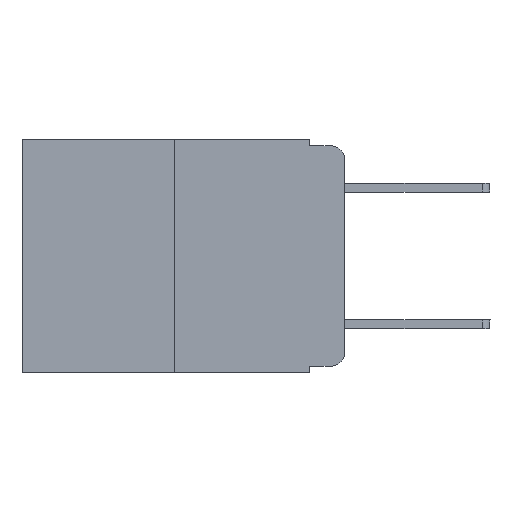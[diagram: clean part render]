
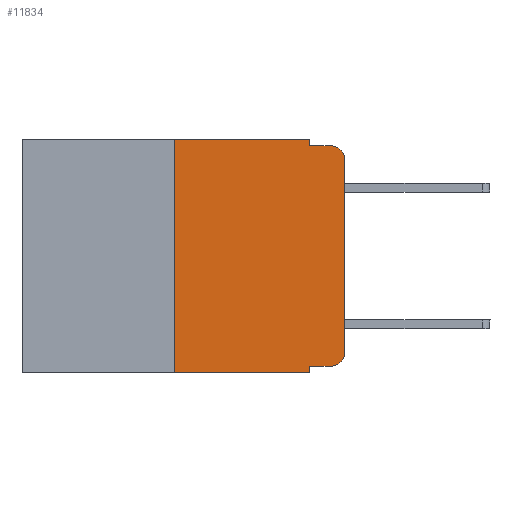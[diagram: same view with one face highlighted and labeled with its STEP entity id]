
A CAD part, left-side view. The second image highlights one B-rep face of the part: STEP entity #11834.
In plain terms, the highlighted planar face has unit normal (-1, 0, 0).
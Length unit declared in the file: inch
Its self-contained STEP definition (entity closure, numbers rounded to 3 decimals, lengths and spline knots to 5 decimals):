
#451 = AXIS2_PLACEMENT_3D ( 'NONE', #14235, #2029, #8772 ) ;
#855 = CARTESIAN_POINT ( 'NONE',  ( 0., 0.473, 0. ) ) ;
#1038 = EDGE_CURVE ( 'NONE', #10655, #8955, #6336, .T. ) ;
#1253 = EDGE_CURVE ( 'NONE', #8012, #3410, #5276, .T. ) ;
#1262 = CARTESIAN_POINT ( 'NONE',  ( 0., 0.051, 0. ) ) ;
#1288 = CARTESIAN_POINT ( 'NONE',  ( 0., 0.02, -0.313 ) ) ;
#1420 = ORIENTED_EDGE ( 'NONE', *, *, #1038, .T. ) ;
#1457 = VERTEX_POINT ( 'NONE', #3869 ) ;
#1613 = ORIENTED_EDGE ( 'NONE', *, *, #9621, .F. ) ;
#1692 = CARTESIAN_POINT ( 'NONE',  ( 0., 0.051, 0. ) ) ;
#1774 = CARTESIAN_POINT ( 'NONE',  ( 0., 0.473, 0. ) ) ;
#1910 = EDGE_CURVE ( 'NONE', #1457, #4394, #10115, .T. ) ;
#2029 = DIRECTION ( 'NONE',  ( -1., 0., 0. ) ) ;
#2167 = AXIS2_PLACEMENT_3D ( 'NONE', #855, #3183, #9697 ) ;
#2798 = VECTOR ( 'NONE', #8173, 39.37008 ) ;
#3183 = DIRECTION ( 'NONE',  ( 1., 0., 0. ) ) ;
#3223 = ORIENTED_EDGE ( 'NONE', *, *, #11476, .T. ) ;
#3271 = VECTOR ( 'NONE', #13562, 39.37008 ) ;
#3306 = ORIENTED_EDGE ( 'NONE', *, *, #6780, .T. ) ;
#3410 = VERTEX_POINT ( 'NONE', #4559 ) ;
#3541 = VECTOR ( 'NONE', #11529, 39.37008 ) ;
#3568 = DIRECTION ( 'NONE',  ( -1., 0., 0. ) ) ;
#3580 = CARTESIAN_POINT ( 'NONE',  ( 0., 0.051, -0.343 ) ) ;
#3869 = CARTESIAN_POINT ( 'NONE',  ( 0., 0.051, -0.01 ) ) ;
#4218 = AXIS2_PLACEMENT_3D ( 'NONE', #1288, #3568, #4650 ) ;
#4323 = CARTESIAN_POINT ( 'NONE',  ( 0., 0.25, 0. ) ) ;
#4394 = VERTEX_POINT ( 'NONE', #11093 ) ;
#4559 = CARTESIAN_POINT ( 'NONE',  ( 0., 0., -0.313 ) ) ;
#4650 = DIRECTION ( 'NONE',  ( 0., 0., -1. ) ) ;
#4877 = CARTESIAN_POINT ( 'NONE',  ( 0., 0., 0. ) ) ;
#5066 = LINE ( 'NONE', #4877, #2798 ) ;
#5276 = CIRCLE ( 'NONE', #4218, 0.02 ) ;
#5320 = CARTESIAN_POINT ( 'NONE',  ( 0., 0.473, -0.343 ) ) ;
#6317 = LINE ( 'NONE', #1774, #8045 ) ;
#6336 = LINE ( 'NONE', #5320, #14302 ) ;
#6348 = ORIENTED_EDGE ( 'NONE', *, *, #8109, .F. ) ;
#6541 = VERTEX_POINT ( 'NONE', #1692 ) ;
#6628 = ORIENTED_EDGE ( 'NONE', *, *, #1253, .T. ) ;
#6654 = ORIENTED_EDGE ( 'NONE', *, *, #8876, .F. ) ;
#6780 = EDGE_CURVE ( 'NONE', #7190, #4394, #12344, .T. ) ;
#6970 = ORIENTED_EDGE ( 'NONE', *, *, #1910, .F. ) ;
#7190 = VERTEX_POINT ( 'NONE', #10620 ) ;
#7437 = ORIENTED_EDGE ( 'NONE', *, *, #13687, .F. ) ;
#7498 = DIRECTION ( 'NONE',  ( 0., -1., 0. ) ) ;
#7536 = PLANE ( 'NONE',  #2167 ) ;
#7747 = ORIENTED_EDGE ( 'NONE', *, *, #14202, .T. ) ;
#7785 = EDGE_LOOP ( 'NONE', ( #7747, #3306, #6970, #6654, #7437, #1613, #1420, #6348, #3223, #6628 ) ) ;
#7915 = DIRECTION ( 'NONE',  ( 0., 0., -1. ) ) ;
#7968 = LINE ( 'NONE', #1262, #8497 ) ;
#8012 = VERTEX_POINT ( 'NONE', #9211 ) ;
#8045 = VECTOR ( 'NONE', #9549, 39.37008 ) ;
#8109 = EDGE_CURVE ( 'NONE', #11433, #8955, #7968, .T. ) ;
#8173 = DIRECTION ( 'NONE',  ( 0., 0., 1. ) ) ;
#8213 = CARTESIAN_POINT ( 'NONE',  ( 0., 0.051, -0.333 ) ) ;
#8447 = LINE ( 'NONE', #4323, #12782 ) ;
#8497 = VECTOR ( 'NONE', #7915, 39.37008 ) ;
#8633 = CARTESIAN_POINT ( 'NONE',  ( 0., 0.25, -0.343 ) ) ;
#8772 = DIRECTION ( 'NONE',  ( 0., 0., -1. ) ) ;
#8876 = EDGE_CURVE ( 'NONE', #6541, #1457, #12963, .T. ) ;
#8955 = VERTEX_POINT ( 'NONE', #3580 ) ;
#9211 = CARTESIAN_POINT ( 'NONE',  ( 0., 0.02, -0.333 ) ) ;
#9267 = VECTOR ( 'NONE', #10403, 39.37008 ) ;
#9549 = DIRECTION ( 'NONE',  ( 0., -1., 0. ) ) ;
#9621 = EDGE_CURVE ( 'NONE', #10655, #11390, #8447, .T. ) ;
#9697 = DIRECTION ( 'NONE',  ( 0., 0., -1. ) ) ;
#10115 = LINE ( 'NONE', #10451, #9267 ) ;
#10403 = DIRECTION ( 'NONE',  ( 0., -1., 0. ) ) ;
#10451 = CARTESIAN_POINT ( 'NONE',  ( 0., 0.051, -0.01 ) ) ;
#10620 = CARTESIAN_POINT ( 'NONE',  ( 0., 0., -0.03 ) ) ;
#10655 = VERTEX_POINT ( 'NONE', #8633 ) ;
#11093 = CARTESIAN_POINT ( 'NONE',  ( 0., 0.02, -0.01 ) ) ;
#11390 = VERTEX_POINT ( 'NONE', #11673 ) ;
#11433 = VERTEX_POINT ( 'NONE', #12605 ) ;
#11476 = EDGE_CURVE ( 'NONE', #11433, #8012, #12552, .T. ) ;
#11529 = DIRECTION ( 'NONE',  ( 0., -1., 0. ) ) ;
#11673 = CARTESIAN_POINT ( 'NONE',  ( 0., 0.25, 0. ) ) ;
#11834 = ADVANCED_FACE ( 'NONE', ( #14159 ), #7536, .F. ) ;
#12064 = DIRECTION ( 'NONE',  ( 0., 0., 1. ) ) ;
#12344 = CIRCLE ( 'NONE', #451, 0.02 ) ;
#12404 = CARTESIAN_POINT ( 'NONE',  ( 0., 0.051, 0. ) ) ;
#12552 = LINE ( 'NONE', #8213, #3541 ) ;
#12605 = CARTESIAN_POINT ( 'NONE',  ( 0., 0.051, -0.333 ) ) ;
#12782 = VECTOR ( 'NONE', #12064, 39.37008 ) ;
#12963 = LINE ( 'NONE', #12404, #3271 ) ;
#13562 = DIRECTION ( 'NONE',  ( 0., 0., -1. ) ) ;
#13687 = EDGE_CURVE ( 'NONE', #11390, #6541, #6317, .T. ) ;
#14159 = FACE_OUTER_BOUND ( 'NONE', #7785, .T. ) ;
#14202 = EDGE_CURVE ( 'NONE', #3410, #7190, #5066, .T. ) ;
#14235 = CARTESIAN_POINT ( 'NONE',  ( 0., 0.02, -0.03 ) ) ;
#14302 = VECTOR ( 'NONE', #7498, 39.37008 ) ;
